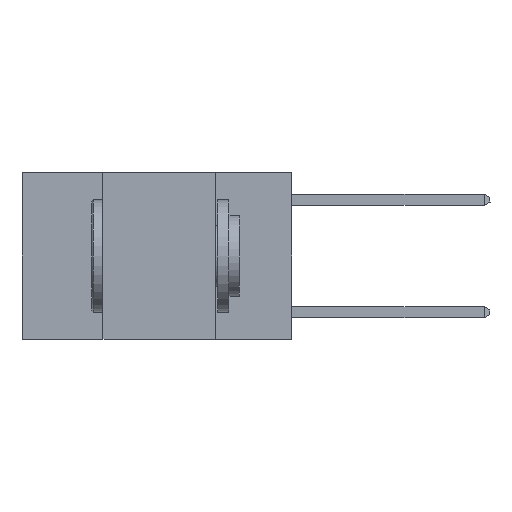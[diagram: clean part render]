
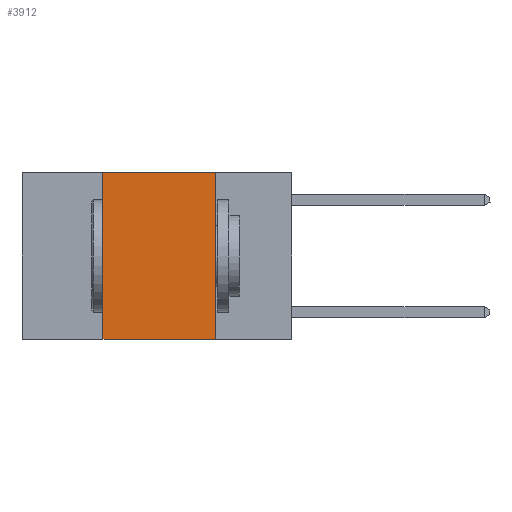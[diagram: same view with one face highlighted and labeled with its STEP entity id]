
A CAD part, left-side view. The second image highlights one B-rep face of the part: STEP entity #3912.
In plain terms, the highlighted planar face has unit normal (-1, 0, 0).
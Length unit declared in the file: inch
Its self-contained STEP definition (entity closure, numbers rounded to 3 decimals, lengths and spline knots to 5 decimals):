
#457 = FACE_OUTER_BOUND ( 'NONE', #8235, .T. ) ;
#512 = ORIENTED_EDGE ( 'NONE', *, *, #3432, .T. ) ;
#851 = ORIENTED_EDGE ( 'NONE', *, *, #3742, .F. ) ;
#1039 = AXIS2_PLACEMENT_3D ( 'NONE', #1051, #6026, #5998 ) ;
#1051 = CARTESIAN_POINT ( 'NONE',  ( 0., 0.6, 0. ) ) ;
#1402 = LINE ( 'NONE', #3638, #1480 ) ;
#1480 = VECTOR ( 'NONE', #3882, 39.37008 ) ;
#1795 = ORIENTED_EDGE ( 'NONE', *, *, #6401, .F. ) ;
#1804 = ORIENTED_EDGE ( 'NONE', *, *, #9559, .F. ) ;
#2380 = CARTESIAN_POINT ( 'NONE',  ( 0., 0.17, 0. ) ) ;
#2575 = CARTESIAN_POINT ( 'NONE',  ( 0., 0.17, -0.37 ) ) ;
#2753 = VECTOR ( 'NONE', #7268, 39.37008 ) ;
#2853 = LINE ( 'NONE', #4939, #2753 ) ;
#3110 = LINE ( 'NONE', #8367, #6934 ) ;
#3432 = EDGE_CURVE ( 'NONE', #5380, #7128, #2853, .T. ) ;
#3638 = CARTESIAN_POINT ( 'NONE',  ( 0., 0.17, 0. ) ) ;
#3742 = EDGE_CURVE ( 'NONE', #5097, #7128, #1402, .T. ) ;
#3752 = CARTESIAN_POINT ( 'NONE',  ( 0., 0.42, 0. ) ) ;
#3882 = DIRECTION ( 'NONE',  ( 0., 0., -1. ) ) ;
#3912 = ADVANCED_FACE ( 'NONE', ( #457 ), #4833, .F. ) ;
#4833 = PLANE ( 'NONE',  #1039 ) ;
#4939 = CARTESIAN_POINT ( 'NONE',  ( 0., 0.6, -0.37 ) ) ;
#5097 = VERTEX_POINT ( 'NONE', #2380 ) ;
#5380 = VERTEX_POINT ( 'NONE', #9579 ) ;
#5413 = VECTOR ( 'NONE', #7379, 39.37008 ) ;
#5648 = VERTEX_POINT ( 'NONE', #3752 ) ;
#5998 = DIRECTION ( 'NONE',  ( 0., 0., -1. ) ) ;
#6026 = DIRECTION ( 'NONE',  ( 1., 0., 0. ) ) ;
#6401 = EDGE_CURVE ( 'NONE', #5648, #5097, #9237, .T. ) ;
#6631 = CARTESIAN_POINT ( 'NONE',  ( 0., 0.6, 0. ) ) ;
#6934 = VECTOR ( 'NONE', #9191, 39.37008 ) ;
#7128 = VERTEX_POINT ( 'NONE', #2575 ) ;
#7268 = DIRECTION ( 'NONE',  ( 0., -1., 0. ) ) ;
#7379 = DIRECTION ( 'NONE',  ( 0., -1., 0. ) ) ;
#8235 = EDGE_LOOP ( 'NONE', ( #851, #1795, #1804, #512 ) ) ;
#8367 = CARTESIAN_POINT ( 'NONE',  ( 0., 0.42, 0. ) ) ;
#9191 = DIRECTION ( 'NONE',  ( 0., 0., 1. ) ) ;
#9237 = LINE ( 'NONE', #6631, #5413 ) ;
#9559 = EDGE_CURVE ( 'NONE', #5380, #5648, #3110, .T. ) ;
#9579 = CARTESIAN_POINT ( 'NONE',  ( 0., 0.42, -0.37 ) ) ;
